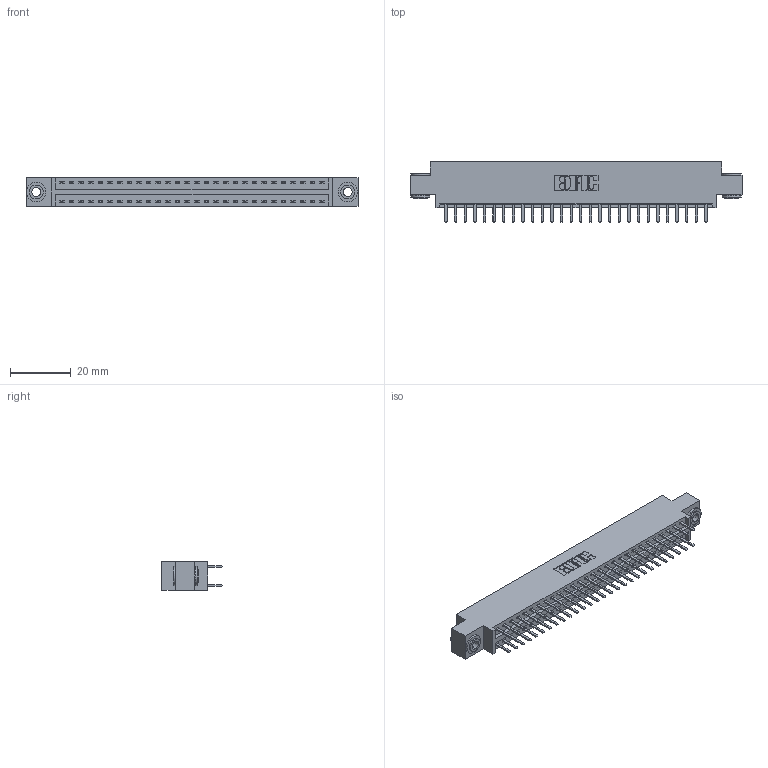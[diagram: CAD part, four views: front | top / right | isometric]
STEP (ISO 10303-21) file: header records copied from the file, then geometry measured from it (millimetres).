
FILE_DESCRIPTION (( 'STEP AP203' ), '1' );
FILE_NAME ('396-056-520-803.STEP', '2019-11-02T08:10:21', ( '' ), ( '' ), 'SwSTEP 2.0', 'SolidWorks 2016', '' );
FILE_SCHEMA (( 'CONFIG_CONTROL_DESIGN' ));
Length unit declared in the file: inch
Products named in the file (4): 346 Part_0.170 Offset - 0.156 Dia-TH; 345-292-001_345-293-120; 345-250-002_345-250-002-102; 396-056-520-803
Assembly tree (59 placements, depth 2):
  396-056-520-803
    346 Part_0.170 Offset - 0.156 Dia-TH
    345-292-001_345-293-120  x56
    345-250-002_345-250-002-102  x2
Bounding box: 109.47 x 20.02 x 9.4 mm (x, y, z)
Volume: 10406.5 mm3; surface area: 14420.5 mm2
Topology: 59 solids, 59 shells, 3300 faces, 9545 edges, 6210 vertices
Faces by surface type: plane 2162, cylinder 1130, cone 8
Entity records: 21054 total; most frequent: CARTESIAN_POINT 3479, ORIENTED_EDGE 3394, DIRECTION 3135, EDGE_CURVE 1697, VECTOR 1425, LINE 1425, VERTEX_POINT 1126, AXIS2_PLACEMENT_3D 855
